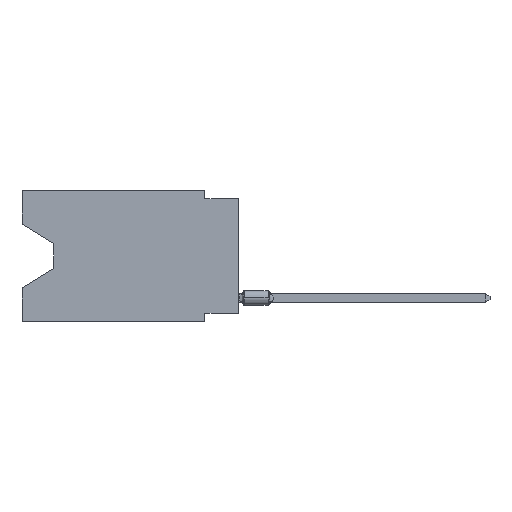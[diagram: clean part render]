
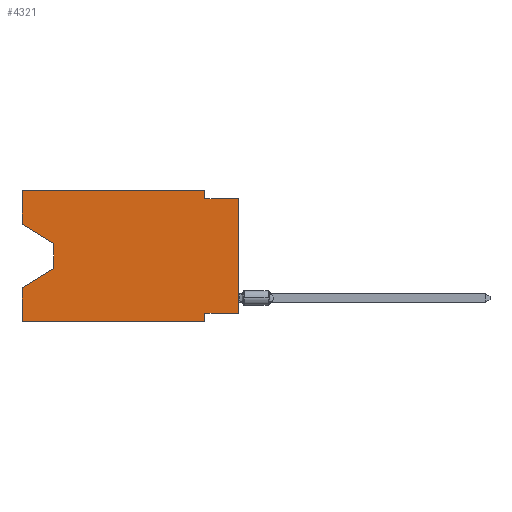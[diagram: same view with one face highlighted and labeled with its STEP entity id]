
A CAD part, left-side view. The second image highlights one B-rep face of the part: STEP entity #4321.
In plain terms, the highlighted planar face has unit normal (-1, 0, 0).
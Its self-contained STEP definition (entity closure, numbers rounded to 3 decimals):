
#59 = DIRECTION ( 'NONE',  ( 1., 0., 0. ) ) ;
#154 = CARTESIAN_POINT ( 'NONE',  ( 0., 16.383, -7.36 ) ) ;
#552 = PLANE ( 'NONE',  #9789 ) ;
#731 = LINE ( 'NONE', #23715, #16591 ) ;
#2015 = VECTOR ( 'NONE', #2707, 1000. ) ;
#2035 = ORIENTED_EDGE ( 'NONE', *, *, #5721, .T. ) ;
#2238 = CARTESIAN_POINT ( 'NONE',  ( 0., 16.383, 0. ) ) ;
#2239 = VERTEX_POINT ( 'NONE', #4225 ) ;
#2279 = EDGE_CURVE ( 'NONE', #19791, #18510, #22640, .T. ) ;
#2616 = VERTEX_POINT ( 'NONE', #13988 ) ;
#2707 = DIRECTION ( 'NONE',  ( 0., 0., -1. ) ) ;
#2729 = DIRECTION ( 'NONE',  ( 0., -1., 0. ) ) ;
#2821 = EDGE_CURVE ( 'NONE', #11528, #18510, #731, .T. ) ;
#3273 = EDGE_CURVE ( 'NONE', #13083, #2616, #21258, .T. ) ;
#3536 = VECTOR ( 'NONE', #11685, 1000. ) ;
#4225 = CARTESIAN_POINT ( 'NONE',  ( 0., 0., -9.271 ) ) ;
#4321 = ADVANCED_FACE ( 'NONE', ( #16533 ), #552, .F. ) ;
#4522 = CARTESIAN_POINT ( 'NONE',  ( 0., 16.383, 0. ) ) ;
#4797 = DIRECTION ( 'NONE',  ( 0., 1., 0. ) ) ;
#4968 = LINE ( 'NONE', #7146, #21908 ) ;
#5418 = DIRECTION ( 'NONE',  ( 0., 0., 1. ) ) ;
#5721 = EDGE_CURVE ( 'NONE', #20649, #17047, #16645, .T. ) ;
#5809 = CARTESIAN_POINT ( 'NONE',  ( 0., 13.97, -5.893 ) ) ;
#5937 = ORIENTED_EDGE ( 'NONE', *, *, #13736, .F. ) ;
#5944 = CARTESIAN_POINT ( 'NONE',  ( 0., 13.97, -4.013 ) ) ;
#5997 = DIRECTION ( 'NONE',  ( 0., -1., 0. ) ) ;
#6301 = ORIENTED_EDGE ( 'NONE', *, *, #22689, .F. ) ;
#6454 = DIRECTION ( 'NONE',  ( 0., -0.855, -0.519 ) ) ;
#7014 = LINE ( 'NONE', #14120, #14762 ) ;
#7137 = VERTEX_POINT ( 'NONE', #12087 ) ;
#7146 = CARTESIAN_POINT ( 'NONE',  ( 0., 0., -0.635 ) ) ;
#7148 = DIRECTION ( 'NONE',  ( 0., 0.855, -0.519 ) ) ;
#9312 = CARTESIAN_POINT ( 'NONE',  ( 0., 16.383, -9.906 ) ) ;
#9371 = ORIENTED_EDGE ( 'NONE', *, *, #15861, .F. ) ;
#9490 = EDGE_CURVE ( 'NONE', #11228, #13083, #11807, .T. ) ;
#9789 = AXIS2_PLACEMENT_3D ( 'NONE', #12928, #59, #16647 ) ;
#9821 = VECTOR ( 'NONE', #11560, 1000. ) ;
#10012 = CARTESIAN_POINT ( 'NONE',  ( 0., 16.383, 0. ) ) ;
#10263 = ORIENTED_EDGE ( 'NONE', *, *, #9490, .F. ) ;
#10463 = VECTOR ( 'NONE', #2729, 1000. ) ;
#10820 = ORIENTED_EDGE ( 'NONE', *, *, #2279, .F. ) ;
#11228 = VERTEX_POINT ( 'NONE', #12601 ) ;
#11327 = CARTESIAN_POINT ( 'NONE',  ( 0., 0., 0. ) ) ;
#11498 = ORIENTED_EDGE ( 'NONE', *, *, #2821, .T. ) ;
#11528 = VERTEX_POINT ( 'NONE', #9312 ) ;
#11560 = DIRECTION ( 'NONE',  ( 0., 0., 1. ) ) ;
#11685 = DIRECTION ( 'NONE',  ( 0., 0., -1. ) ) ;
#11807 = LINE ( 'NONE', #10012, #9821 ) ;
#11824 = VERTEX_POINT ( 'NONE', #16140 ) ;
#12087 = CARTESIAN_POINT ( 'NONE',  ( 0., 2.54, -0.635 ) ) ;
#12191 = VECTOR ( 'NONE', #7148, 1000. ) ;
#12274 = EDGE_CURVE ( 'NONE', #2239, #11824, #18544, .T. ) ;
#12524 = CARTESIAN_POINT ( 'NONE',  ( 0., 16.383, 0. ) ) ;
#12601 = CARTESIAN_POINT ( 'NONE',  ( 0., 16.383, -2.546 ) ) ;
#12928 = CARTESIAN_POINT ( 'NONE',  ( 0., 16.383, 0. ) ) ;
#12975 = ORIENTED_EDGE ( 'NONE', *, *, #21739, .F. ) ;
#13083 = VERTEX_POINT ( 'NONE', #2238 ) ;
#13145 = ORIENTED_EDGE ( 'NONE', *, *, #16500, .T. ) ;
#13736 = EDGE_CURVE ( 'NONE', #11528, #17047, #21668, .T. ) ;
#13949 = LINE ( 'NONE', #21305, #21316 ) ;
#13988 = CARTESIAN_POINT ( 'NONE',  ( 0., 2.54, 0. ) ) ;
#14035 = CARTESIAN_POINT ( 'NONE',  ( 0., 16.383, -2.546 ) ) ;
#14120 = CARTESIAN_POINT ( 'NONE',  ( 0., 2.54, 0. ) ) ;
#14486 = DIRECTION ( 'NONE',  ( 0., -1., 0. ) ) ;
#14762 = VECTOR ( 'NONE', #21461, 1000. ) ;
#15601 = LINE ( 'NONE', #14035, #17875 ) ;
#15648 = VERTEX_POINT ( 'NONE', #5944 ) ;
#15861 = EDGE_CURVE ( 'NONE', #2616, #7137, #7014, .T. ) ;
#15892 = DIRECTION ( 'NONE',  ( 0., 0., 1. ) ) ;
#15928 = LINE ( 'NONE', #19087, #2015 ) ;
#16140 = CARTESIAN_POINT ( 'NONE',  ( 0., 0., -0.635 ) ) ;
#16500 = EDGE_CURVE ( 'NONE', #11228, #15648, #15601, .T. ) ;
#16533 = FACE_OUTER_BOUND ( 'NONE', #19095, .T. ) ;
#16591 = VECTOR ( 'NONE', #5997, 1000. ) ;
#16645 = LINE ( 'NONE', #5809, #12191 ) ;
#16647 = DIRECTION ( 'NONE',  ( 0., 0., -1. ) ) ;
#16837 = EDGE_CURVE ( 'NONE', #15648, #20649, #15928, .T. ) ;
#16936 = CARTESIAN_POINT ( 'NONE',  ( 0., 13.97, -5.893 ) ) ;
#16985 = CARTESIAN_POINT ( 'NONE',  ( 0., 2.54, -9.906 ) ) ;
#17047 = VERTEX_POINT ( 'NONE', #154 ) ;
#17875 = VECTOR ( 'NONE', #6454, 1000. ) ;
#18373 = ORIENTED_EDGE ( 'NONE', *, *, #16837, .T. ) ;
#18510 = VERTEX_POINT ( 'NONE', #20854 ) ;
#18544 = LINE ( 'NONE', #11327, #23009 ) ;
#19087 = CARTESIAN_POINT ( 'NONE',  ( 0., 13.97, -4.013 ) ) ;
#19095 = EDGE_LOOP ( 'NONE', ( #13145, #18373, #2035, #5937, #11498, #10820, #12975, #19725, #6301, #9371, #20241, #10263 ) ) ;
#19725 = ORIENTED_EDGE ( 'NONE', *, *, #12274, .T. ) ;
#19791 = VERTEX_POINT ( 'NONE', #20611 ) ;
#20241 = ORIENTED_EDGE ( 'NONE', *, *, #3273, .F. ) ;
#20611 = CARTESIAN_POINT ( 'NONE',  ( 0., 2.54, -9.271 ) ) ;
#20649 = VERTEX_POINT ( 'NONE', #16936 ) ;
#20854 = CARTESIAN_POINT ( 'NONE',  ( 0., 2.54, -9.906 ) ) ;
#21258 = LINE ( 'NONE', #4522, #10463 ) ;
#21305 = CARTESIAN_POINT ( 'NONE',  ( 0., 0., -9.271 ) ) ;
#21316 = VECTOR ( 'NONE', #4797, 1000. ) ;
#21361 = VECTOR ( 'NONE', #15892, 1000. ) ;
#21461 = DIRECTION ( 'NONE',  ( 0., 0., -1. ) ) ;
#21668 = LINE ( 'NONE', #12524, #21361 ) ;
#21739 = EDGE_CURVE ( 'NONE', #2239, #19791, #13949, .T. ) ;
#21908 = VECTOR ( 'NONE', #14486, 1000. ) ;
#22640 = LINE ( 'NONE', #16985, #3536 ) ;
#22689 = EDGE_CURVE ( 'NONE', #7137, #11824, #4968, .T. ) ;
#23009 = VECTOR ( 'NONE', #5418, 1000. ) ;
#23715 = CARTESIAN_POINT ( 'NONE',  ( 0., 16.383, -9.906 ) ) ;
